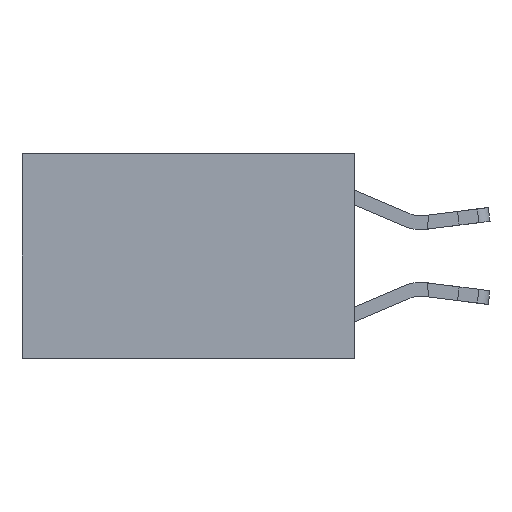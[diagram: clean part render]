
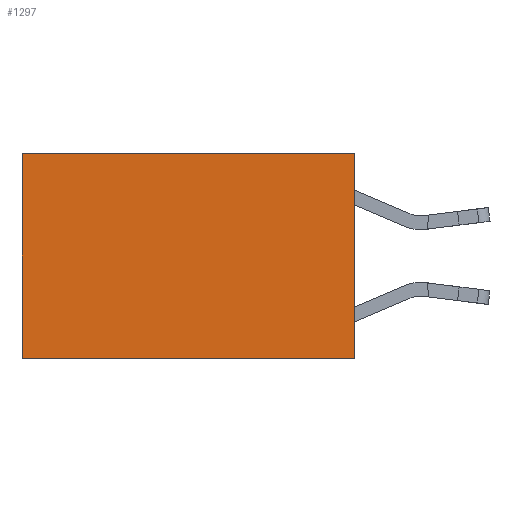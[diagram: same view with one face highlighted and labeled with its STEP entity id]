
A CAD part, left-side view. The second image highlights one B-rep face of the part: STEP entity #1297.
In plain terms, the highlighted planar face has unit normal (-1, 0, 0).
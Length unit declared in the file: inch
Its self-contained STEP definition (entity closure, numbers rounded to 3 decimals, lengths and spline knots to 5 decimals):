
#327 = ORIENTED_EDGE ( 'NONE', *, *, #6748, .T. ) ;
#348 = CARTESIAN_POINT ( 'NONE',  ( 0.2625, 0.6, 0. ) ) ;
#519 = LINE ( 'NONE', #5379, #6158 ) ;
#748 = EDGE_LOOP ( 'NONE', ( #2562, #1783, #11254, #327 ) ) ;
#959 = LINE ( 'NONE', #348, #6972 ) ;
#977 = VECTOR ( 'NONE', #11294, 39.37008 ) ;
#1206 = LINE ( 'NONE', #4101, #12443 ) ;
#1297 = ADVANCED_FACE ( 'NONE', ( #10077 ), #4360, .F. ) ;
#1471 = EDGE_CURVE ( 'NONE', #5881, #3103, #11617, .T. ) ;
#1755 = EDGE_CURVE ( 'NONE', #3084, #3103, #959, .T. ) ;
#1783 = ORIENTED_EDGE ( 'NONE', *, *, #1471, .F. ) ;
#1862 = CARTESIAN_POINT ( 'NONE',  ( 0.2625, 0.6, -0.37 ) ) ;
#1939 = DIRECTION ( 'NONE',  ( 0., 0., -1. ) ) ;
#2562 = ORIENTED_EDGE ( 'NONE', *, *, #1755, .T. ) ;
#3084 = VERTEX_POINT ( 'NONE', #9604 ) ;
#3103 = VERTEX_POINT ( 'NONE', #1862 ) ;
#3598 = VERTEX_POINT ( 'NONE', #7595 ) ;
#3769 = CARTESIAN_POINT ( 'NONE',  ( 0.2625, 0., -0.37 ) ) ;
#4101 = CARTESIAN_POINT ( 'NONE',  ( 0.2625, 0., 0. ) ) ;
#4360 = PLANE ( 'NONE',  #12852 ) ;
#4473 = CARTESIAN_POINT ( 'NONE',  ( 0.2625, 0., 0. ) ) ;
#5379 = CARTESIAN_POINT ( 'NONE',  ( 0.2625, 0., 0. ) ) ;
#5881 = VERTEX_POINT ( 'NONE', #3769 ) ;
#6158 = VECTOR ( 'NONE', #1939, 39.37008 ) ;
#6348 = DIRECTION ( 'NONE',  ( 0., 1., 0. ) ) ;
#6748 = EDGE_CURVE ( 'NONE', #3598, #3084, #1206, .T. ) ;
#6836 = EDGE_CURVE ( 'NONE', #3598, #5881, #519, .T. ) ;
#6972 = VECTOR ( 'NONE', #12003, 39.37008 ) ;
#7595 = CARTESIAN_POINT ( 'NONE',  ( 0.2625, 0., 0. ) ) ;
#7709 = DIRECTION ( 'NONE',  ( 0., 0., -1. ) ) ;
#8008 = DIRECTION ( 'NONE',  ( 1., 0., 0. ) ) ;
#9571 = CARTESIAN_POINT ( 'NONE',  ( 0.2625, 0., -0.37 ) ) ;
#9604 = CARTESIAN_POINT ( 'NONE',  ( 0.2625, 0.6, 0. ) ) ;
#10077 = FACE_OUTER_BOUND ( 'NONE', #748, .T. ) ;
#11254 = ORIENTED_EDGE ( 'NONE', *, *, #6836, .F. ) ;
#11294 = DIRECTION ( 'NONE',  ( 0., 1., 0. ) ) ;
#11617 = LINE ( 'NONE', #9571, #977 ) ;
#12003 = DIRECTION ( 'NONE',  ( 0., 0., -1. ) ) ;
#12443 = VECTOR ( 'NONE', #6348, 39.37008 ) ;
#12852 = AXIS2_PLACEMENT_3D ( 'NONE', #4473, #8008, #7709 ) ;
